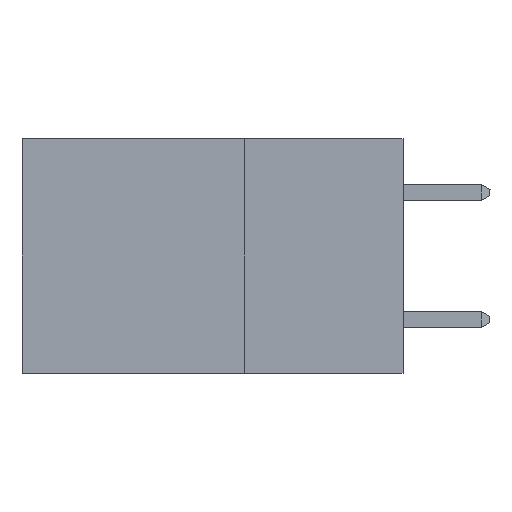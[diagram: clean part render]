
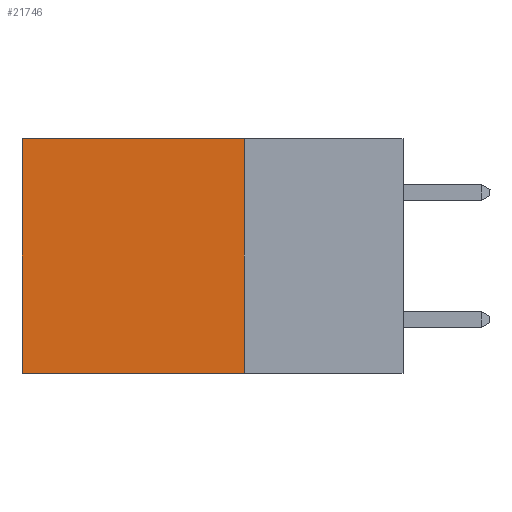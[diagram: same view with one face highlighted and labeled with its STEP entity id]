
A CAD part, left-side view. The second image highlights one B-rep face of the part: STEP entity #21746.
In plain terms, the highlighted planar face has unit normal (-1, 0, 0).
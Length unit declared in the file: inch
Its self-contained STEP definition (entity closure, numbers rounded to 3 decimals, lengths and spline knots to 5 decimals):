
#372 = LINE ( 'NONE', #15857, #16289 ) ;
#624 = DIRECTION ( 'NONE',  ( 0., 1., 0. ) ) ;
#1327 = DIRECTION ( 'NONE',  ( 0., 0., -1. ) ) ;
#1684 = DIRECTION ( 'NONE',  ( 1., 0., 0. ) ) ;
#2399 = LINE ( 'NONE', #8124, #13499 ) ;
#2464 = ORIENTED_EDGE ( 'NONE', *, *, #7624, .F. ) ;
#4001 = FACE_OUTER_BOUND ( 'NONE', #15301, .T. ) ;
#4625 = CARTESIAN_POINT ( 'NONE',  ( 0.2875, 0.25, -0.37 ) ) ;
#4914 = VERTEX_POINT ( 'NONE', #19838 ) ;
#5461 = LINE ( 'NONE', #10703, #26479 ) ;
#6183 = LINE ( 'NONE', #25185, #16580 ) ;
#6880 = ORIENTED_EDGE ( 'NONE', *, *, #7089, .F. ) ;
#7089 = EDGE_CURVE ( 'NONE', #19023, #19319, #5461, .T. ) ;
#7624 = EDGE_CURVE ( 'NONE', #4914, #19023, #2399, .T. ) ;
#8124 = CARTESIAN_POINT ( 'NONE',  ( 0.2875, 0.25, 0. ) ) ;
#10166 = CARTESIAN_POINT ( 'NONE',  ( 0.2875, 0.6, -0.37 ) ) ;
#10211 = DIRECTION ( 'NONE',  ( 0., 0., -1. ) ) ;
#10703 = CARTESIAN_POINT ( 'NONE',  ( 0.2875, 0.25, -0.37 ) ) ;
#12070 = CARTESIAN_POINT ( 'NONE',  ( 0.2875, 0.6, 0. ) ) ;
#12822 = DIRECTION ( 'NONE',  ( 0., 1., 0. ) ) ;
#12942 = AXIS2_PLACEMENT_3D ( 'NONE', #14138, #1684, #16208 ) ;
#13499 = VECTOR ( 'NONE', #10211, 39.37008 ) ;
#14138 = CARTESIAN_POINT ( 'NONE',  ( 0.2875, 0.25, 0. ) ) ;
#15301 = EDGE_LOOP ( 'NONE', ( #25427, #6880, #2464, #24930 ) ) ;
#15755 = EDGE_CURVE ( 'NONE', #4914, #19927, #6183, .T. ) ;
#15857 = CARTESIAN_POINT ( 'NONE',  ( 0.2875, 0.6, 0. ) ) ;
#16208 = DIRECTION ( 'NONE',  ( 0., 0., -1. ) ) ;
#16289 = VECTOR ( 'NONE', #1327, 39.37008 ) ;
#16580 = VECTOR ( 'NONE', #624, 39.37008 ) ;
#19023 = VERTEX_POINT ( 'NONE', #4625 ) ;
#19319 = VERTEX_POINT ( 'NONE', #10166 ) ;
#19838 = CARTESIAN_POINT ( 'NONE',  ( 0.2875, 0.25, 0. ) ) ;
#19927 = VERTEX_POINT ( 'NONE', #12070 ) ;
#21746 = ADVANCED_FACE ( 'NONE', ( #4001 ), #26171, .F. ) ;
#23716 = EDGE_CURVE ( 'NONE', #19927, #19319, #372, .T. ) ;
#24930 = ORIENTED_EDGE ( 'NONE', *, *, #15755, .T. ) ;
#25185 = CARTESIAN_POINT ( 'NONE',  ( 0.2875, 0.25, 0. ) ) ;
#25427 = ORIENTED_EDGE ( 'NONE', *, *, #23716, .T. ) ;
#26171 = PLANE ( 'NONE',  #12942 ) ;
#26479 = VECTOR ( 'NONE', #12822, 39.37008 ) ;
